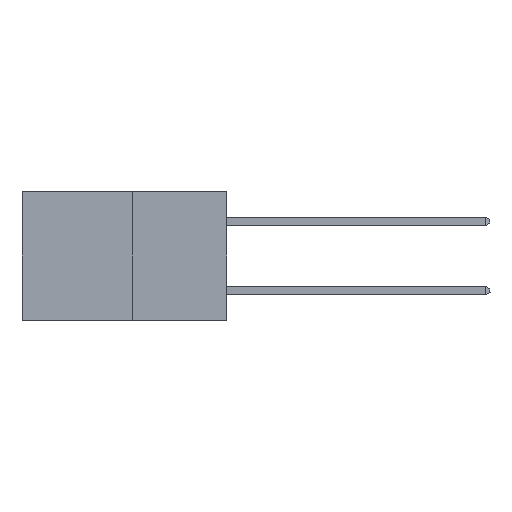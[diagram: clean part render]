
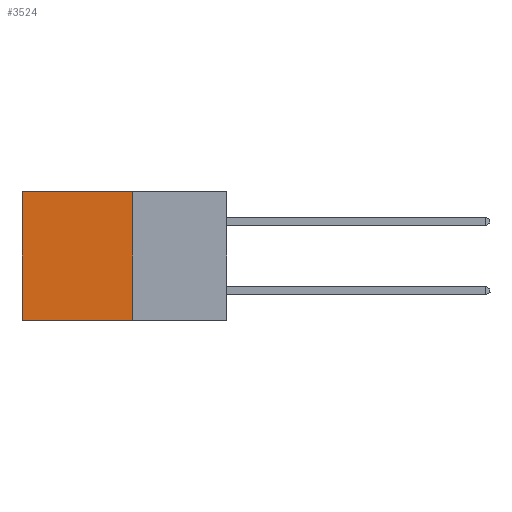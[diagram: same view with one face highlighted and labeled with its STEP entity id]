
A CAD part, left-side view. The second image highlights one B-rep face of the part: STEP entity #3524.
In plain terms, the highlighted planar face has unit normal (-1, 0, 0).
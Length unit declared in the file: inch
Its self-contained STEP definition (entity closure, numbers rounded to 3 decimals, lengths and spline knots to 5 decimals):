
#244 = VECTOR ( 'NONE', #7339, 39.37008 ) ;
#445 = CARTESIAN_POINT ( 'NONE',  ( 0.277, 0.59, -0.37 ) ) ;
#471 = LINE ( 'NONE', #9757, #6985 ) ;
#1713 = VECTOR ( 'NONE', #7893, 39.37008 ) ;
#2247 = ORIENTED_EDGE ( 'NONE', *, *, #2813, .T. ) ;
#2539 = CARTESIAN_POINT ( 'NONE',  ( 0.277, 0.59, 0. ) ) ;
#2813 = EDGE_CURVE ( 'NONE', #3875, #11363, #11719, .T. ) ;
#3393 = DIRECTION ( 'NONE',  ( 0., 0., -1. ) ) ;
#3427 = DIRECTION ( 'NONE',  ( 1., 0., 0. ) ) ;
#3524 = ADVANCED_FACE ( 'NONE', ( #14902 ), #9510, .F. ) ;
#3583 = CARTESIAN_POINT ( 'NONE',  ( 0.277, 0.27, -0.37 ) ) ;
#3633 = DIRECTION ( 'NONE',  ( 0., 1., 0. ) ) ;
#3716 = LINE ( 'NONE', #7643, #244 ) ;
#3875 = VERTEX_POINT ( 'NONE', #2539 ) ;
#4914 = VECTOR ( 'NONE', #3633, 39.37008 ) ;
#5132 = EDGE_CURVE ( 'NONE', #14228, #3875, #471, .T. ) ;
#5793 = ORIENTED_EDGE ( 'NONE', *, *, #5132, .T. ) ;
#6259 = EDGE_CURVE ( 'NONE', #14228, #12660, #3716, .T. ) ;
#6626 = EDGE_CURVE ( 'NONE', #12660, #11363, #15671, .T. ) ;
#6848 = CARTESIAN_POINT ( 'NONE',  ( 0.277, 0.59, -0.37 ) ) ;
#6985 = VECTOR ( 'NONE', #9356, 39.37008 ) ;
#7339 = DIRECTION ( 'NONE',  ( 0., 0., -1. ) ) ;
#7460 = ORIENTED_EDGE ( 'NONE', *, *, #6259, .F. ) ;
#7643 = CARTESIAN_POINT ( 'NONE',  ( 0.277, 0.27, -0.37 ) ) ;
#7893 = DIRECTION ( 'NONE',  ( 0., 0., -1. ) ) ;
#9356 = DIRECTION ( 'NONE',  ( 0., 1., 0. ) ) ;
#9510 = PLANE ( 'NONE',  #11148 ) ;
#9532 = CARTESIAN_POINT ( 'NONE',  ( 0.277, 0.27, -0.37 ) ) ;
#9757 = CARTESIAN_POINT ( 'NONE',  ( 0.277, 0.27, 0. ) ) ;
#10706 = EDGE_LOOP ( 'NONE', ( #2247, #16765, #7460, #5793 ) ) ;
#10757 = CARTESIAN_POINT ( 'NONE',  ( 0.277, 0.27, -0.37 ) ) ;
#11148 = AXIS2_PLACEMENT_3D ( 'NONE', #9532, #3427, #3393 ) ;
#11363 = VERTEX_POINT ( 'NONE', #445 ) ;
#11719 = LINE ( 'NONE', #6848, #1713 ) ;
#12660 = VERTEX_POINT ( 'NONE', #10757 ) ;
#14228 = VERTEX_POINT ( 'NONE', #16574 ) ;
#14902 = FACE_OUTER_BOUND ( 'NONE', #10706, .T. ) ;
#15671 = LINE ( 'NONE', #3583, #4914 ) ;
#16574 = CARTESIAN_POINT ( 'NONE',  ( 0.277, 0.27, 0. ) ) ;
#16765 = ORIENTED_EDGE ( 'NONE', *, *, #6626, .F. ) ;
